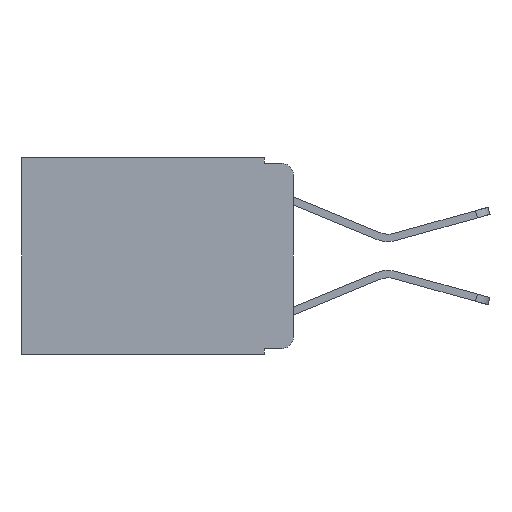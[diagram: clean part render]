
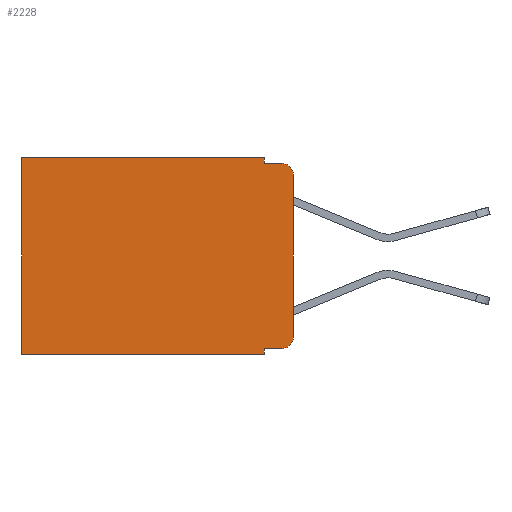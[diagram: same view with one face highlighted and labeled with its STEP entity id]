
A CAD part, left-side view. The second image highlights one B-rep face of the part: STEP entity #2228.
In plain terms, the highlighted planar face has unit normal (-1, 0, 0).
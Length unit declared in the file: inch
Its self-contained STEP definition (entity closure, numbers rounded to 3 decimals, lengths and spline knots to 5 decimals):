
#811 = DIRECTION ( 'NONE',  ( 0., 0., -1. ) ) ;
#905 = VERTEX_POINT ( 'NONE', #13725 ) ;
#996 = EDGE_CURVE ( 'NONE', #11316, #17225, #15752, .T. ) ;
#1151 = VERTEX_POINT ( 'NONE', #5196 ) ;
#1716 = CARTESIAN_POINT ( 'NONE',  ( 0.298, 0.051, 0. ) ) ;
#1770 = VERTEX_POINT ( 'NONE', #1716 ) ;
#1901 = DIRECTION ( 'NONE',  ( -1., 0., 0. ) ) ;
#2228 = ADVANCED_FACE ( 'NONE', ( #10948 ), #11612, .F. ) ;
#2542 = ORIENTED_EDGE ( 'NONE', *, *, #2664, .T. ) ;
#2664 = EDGE_CURVE ( 'NONE', #1151, #7013, #10924, .T. ) ;
#3062 = DIRECTION ( 'NONE',  ( 0., 0., -1. ) ) ;
#3111 = CARTESIAN_POINT ( 'NONE',  ( 0.298, 0.02, -0.333 ) ) ;
#3232 = EDGE_CURVE ( 'NONE', #1770, #14486, #8557, .T. ) ;
#3295 = LINE ( 'NONE', #17880, #12063 ) ;
#3696 = VERTEX_POINT ( 'NONE', #3111 ) ;
#3718 = CARTESIAN_POINT ( 'NONE',  ( 0.298, 0.051, 0. ) ) ;
#4015 = CARTESIAN_POINT ( 'NONE',  ( 0.298, 0.02, -0.01 ) ) ;
#4546 = VERTEX_POINT ( 'NONE', #9617 ) ;
#4758 = DIRECTION ( 'NONE',  ( 0., 0., -1. ) ) ;
#5196 = CARTESIAN_POINT ( 'NONE',  ( 0.298, 0., -0.03 ) ) ;
#5517 = DIRECTION ( 'NONE',  ( 0., 0., -1. ) ) ;
#5542 = ORIENTED_EDGE ( 'NONE', *, *, #996, .F. ) ;
#6650 = VECTOR ( 'NONE', #10149, 39.37008 ) ;
#7013 = VERTEX_POINT ( 'NONE', #4015 ) ;
#7483 = ORIENTED_EDGE ( 'NONE', *, *, #9717, .T. ) ;
#8330 = VECTOR ( 'NONE', #4758, 39.37008 ) ;
#8347 = DIRECTION ( 'NONE',  ( 0., -1., 0. ) ) ;
#8557 = LINE ( 'NONE', #10198, #17015 ) ;
#8609 = VECTOR ( 'NONE', #8347, 39.37008 ) ;
#9029 = DIRECTION ( 'NONE',  ( -1., 0., 0. ) ) ;
#9172 = CARTESIAN_POINT ( 'NONE',  ( 0.298, 0.051, -0.343 ) ) ;
#9617 = CARTESIAN_POINT ( 'NONE',  ( 0.298, 0., -0.313 ) ) ;
#9717 = EDGE_CURVE ( 'NONE', #17290, #3696, #18123, .T. ) ;
#10149 = DIRECTION ( 'NONE',  ( 0., 1., 0. ) ) ;
#10185 = EDGE_CURVE ( 'NONE', #905, #7013, #3295, .T. ) ;
#10198 = CARTESIAN_POINT ( 'NONE',  ( 0.298, 0., 0. ) ) ;
#10295 = CARTESIAN_POINT ( 'NONE',  ( 0.298, 0.473, -0.343 ) ) ;
#10357 = DIRECTION ( 'NONE',  ( 1., 0., 0. ) ) ;
#10924 = CIRCLE ( 'NONE', #19449, 0.02 ) ;
#10948 = FACE_OUTER_BOUND ( 'NONE', #21326, .T. ) ;
#11126 = DIRECTION ( 'NONE',  ( 0., -1., 0. ) ) ;
#11316 = VERTEX_POINT ( 'NONE', #9172 ) ;
#11612 = PLANE ( 'NONE',  #13142 ) ;
#11729 = CARTESIAN_POINT ( 'NONE',  ( 0.298, 0., 0. ) ) ;
#11731 = AXIS2_PLACEMENT_3D ( 'NONE', #19117, #9029, #20755 ) ;
#12043 = ORIENTED_EDGE ( 'NONE', *, *, #10185, .F. ) ;
#12063 = VECTOR ( 'NONE', #11126, 39.37008 ) ;
#12099 = CARTESIAN_POINT ( 'NONE',  ( 0.298, 0.051, -0.333 ) ) ;
#12109 = VECTOR ( 'NONE', #3062, 39.37008 ) ;
#12194 = VECTOR ( 'NONE', #5517, 39.37008 ) ;
#12865 = LINE ( 'NONE', #11729, #8330 ) ;
#13142 = AXIS2_PLACEMENT_3D ( 'NONE', #22160, #10357, #18264 ) ;
#13161 = VECTOR ( 'NONE', #19498, 39.37008 ) ;
#13625 = ORIENTED_EDGE ( 'NONE', *, *, #13728, .F. ) ;
#13725 = CARTESIAN_POINT ( 'NONE',  ( 0.298, 0.051, -0.01 ) ) ;
#13728 = EDGE_CURVE ( 'NONE', #17290, #11316, #16656, .T. ) ;
#13876 = ORIENTED_EDGE ( 'NONE', *, *, #20538, .T. ) ;
#14486 = VERTEX_POINT ( 'NONE', #15284 ) ;
#14693 = ORIENTED_EDGE ( 'NONE', *, *, #3232, .T. ) ;
#15198 = CARTESIAN_POINT ( 'NONE',  ( 0.298, 0.051, 0. ) ) ;
#15225 = ORIENTED_EDGE ( 'NONE', *, *, #18907, .F. ) ;
#15245 = ORIENTED_EDGE ( 'NONE', *, *, #19487, .F. ) ;
#15284 = CARTESIAN_POINT ( 'NONE',  ( 0.298, 0.473, 0. ) ) ;
#15752 = LINE ( 'NONE', #17140, #6650 ) ;
#16656 = LINE ( 'NONE', #3718, #12194 ) ;
#16756 = CARTESIAN_POINT ( 'NONE',  ( 0.298, 0.02, -0.03 ) ) ;
#17015 = VECTOR ( 'NONE', #20215, 39.37008 ) ;
#17140 = CARTESIAN_POINT ( 'NONE',  ( 0.298, 0., -0.343 ) ) ;
#17225 = VERTEX_POINT ( 'NONE', #10295 ) ;
#17290 = VERTEX_POINT ( 'NONE', #12099 ) ;
#17880 = CARTESIAN_POINT ( 'NONE',  ( 0.298, 0.051, -0.01 ) ) ;
#17914 = CARTESIAN_POINT ( 'NONE',  ( 0.298, 0.473, 0. ) ) ;
#18123 = LINE ( 'NONE', #20106, #8609 ) ;
#18264 = DIRECTION ( 'NONE',  ( 0., 0., -1. ) ) ;
#18907 = EDGE_CURVE ( 'NONE', #1770, #905, #20437, .T. ) ;
#19117 = CARTESIAN_POINT ( 'NONE',  ( 0.298, 0.02, -0.313 ) ) ;
#19366 = CIRCLE ( 'NONE', #11731, 0.02 ) ;
#19449 = AXIS2_PLACEMENT_3D ( 'NONE', #16756, #1901, #811 ) ;
#19487 = EDGE_CURVE ( 'NONE', #1151, #4546, #12865, .T. ) ;
#19498 = DIRECTION ( 'NONE',  ( 0., 0., -1. ) ) ;
#20106 = CARTESIAN_POINT ( 'NONE',  ( 0.298, 0.051, -0.333 ) ) ;
#20215 = DIRECTION ( 'NONE',  ( 0., 1., 0. ) ) ;
#20437 = LINE ( 'NONE', #15198, #12109 ) ;
#20538 = EDGE_CURVE ( 'NONE', #3696, #4546, #19366, .T. ) ;
#20755 = DIRECTION ( 'NONE',  ( 0., 0., -1. ) ) ;
#21326 = EDGE_LOOP ( 'NONE', ( #15245, #2542, #12043, #15225, #14693, #21437, #5542, #13625, #7483, #13876 ) ) ;
#21437 = ORIENTED_EDGE ( 'NONE', *, *, #21894, .T. ) ;
#21894 = EDGE_CURVE ( 'NONE', #14486, #17225, #21968, .T. ) ;
#21968 = LINE ( 'NONE', #17914, #13161 ) ;
#22160 = CARTESIAN_POINT ( 'NONE',  ( 0.298, 0., 0. ) ) ;
